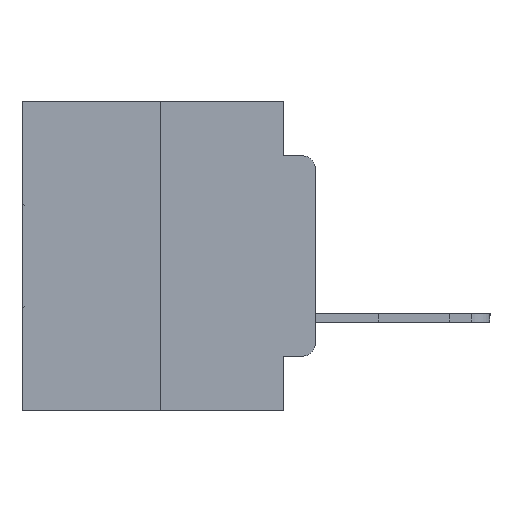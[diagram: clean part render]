
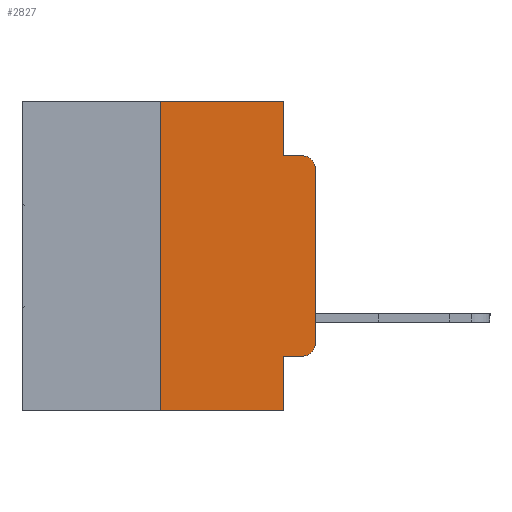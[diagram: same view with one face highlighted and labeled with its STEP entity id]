
A CAD part, left-side view. The second image highlights one B-rep face of the part: STEP entity #2827.
In plain terms, the highlighted planar face has unit normal (-1, 0, 0).
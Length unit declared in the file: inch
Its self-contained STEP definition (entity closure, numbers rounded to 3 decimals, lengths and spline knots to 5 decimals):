
#134 = CIRCLE ( 'NONE', #27930, 0.02 ) ;
#1123 = ORIENTED_EDGE ( 'NONE', *, *, #8856, .T. ) ;
#1332 = DIRECTION ( 'NONE',  ( 0., -1., 0. ) ) ;
#1491 = EDGE_CURVE ( 'NONE', #13249, #27975, #21771, .T. ) ;
#1554 = ORIENTED_EDGE ( 'NONE', *, *, #29062, .F. ) ;
#1798 = DIRECTION ( 'NONE',  ( 0., 0., -1. ) ) ;
#2827 = ADVANCED_FACE ( 'NONE', ( #18176 ), #4792, .F. ) ;
#3279 = EDGE_CURVE ( 'NONE', #28406, #4622, #22686, .T. ) ;
#3371 = CARTESIAN_POINT ( 'NONE',  ( 0., 0.051, 0. ) ) ;
#3413 = VECTOR ( 'NONE', #17441, 39.37008 ) ;
#3831 = VERTEX_POINT ( 'NONE', #18036 ) ;
#4171 = LINE ( 'NONE', #3371, #3413 ) ;
#4533 = CARTESIAN_POINT ( 'NONE',  ( 0., 0.25, 0. ) ) ;
#4622 = VERTEX_POINT ( 'NONE', #25711 ) ;
#4792 = PLANE ( 'NONE',  #17398 ) ;
#4821 = CARTESIAN_POINT ( 'NONE',  ( 0., 0.473, 0. ) ) ;
#4843 = EDGE_CURVE ( 'NONE', #28406, #24494, #4919, .T. ) ;
#4919 = LINE ( 'NONE', #4533, #10415 ) ;
#5857 = DIRECTION ( 'NONE',  ( 0., 0., -1. ) ) ;
#5871 = EDGE_CURVE ( 'NONE', #24494, #3831, #19081, .T. ) ;
#6150 = CARTESIAN_POINT ( 'NONE',  ( 0., 0.051, -0.4115 ) ) ;
#6652 = VECTOR ( 'NONE', #1332, 39.37008 ) ;
#7190 = DIRECTION ( 'NONE',  ( 0., -1., 0. ) ) ;
#7559 = ORIENTED_EDGE ( 'NONE', *, *, #9175, .T. ) ;
#7851 = DIRECTION ( 'NONE',  ( 0., 0., -1. ) ) ;
#7856 = DIRECTION ( 'NONE',  ( 1., 0., 0. ) ) ;
#8427 = LINE ( 'NONE', #21942, #13953 ) ;
#8856 = EDGE_CURVE ( 'NONE', #27269, #22256, #16182, .T. ) ;
#8903 = CARTESIAN_POINT ( 'NONE',  ( 0., 0., -0.3915 ) ) ;
#9065 = LINE ( 'NONE', #24958, #26474 ) ;
#9175 = EDGE_CURVE ( 'NONE', #22256, #16949, #134, .T. ) ;
#10415 = VECTOR ( 'NONE', #26581, 39.37008 ) ;
#10465 = VECTOR ( 'NONE', #12939, 39.37008 ) ;
#10766 = EDGE_CURVE ( 'NONE', #27975, #27269, #16026, .T. ) ;
#10768 = CARTESIAN_POINT ( 'NONE',  ( 0., 0.02, -0.3915 ) ) ;
#12939 = DIRECTION ( 'NONE',  ( 0., -1., 0. ) ) ;
#13145 = DIRECTION ( 'NONE',  ( 0., 0., -1. ) ) ;
#13249 = VERTEX_POINT ( 'NONE', #20065 ) ;
#13715 = DIRECTION ( 'NONE',  ( 0., -1., 0. ) ) ;
#13953 = VECTOR ( 'NONE', #5857, 39.37008 ) ;
#14979 = VECTOR ( 'NONE', #7190, 39.37008 ) ;
#15640 = ORIENTED_EDGE ( 'NONE', *, *, #1491, .T. ) ;
#15964 = CARTESIAN_POINT ( 'NONE',  ( 0., 0.02, -0.1085 ) ) ;
#16026 = CIRCLE ( 'NONE', #27968, 0.02 ) ;
#16182 = LINE ( 'NONE', #19670, #22228 ) ;
#16949 = VERTEX_POINT ( 'NONE', #23699 ) ;
#17398 = AXIS2_PLACEMENT_3D ( 'NONE', #4821, #7856, #7851 ) ;
#17441 = DIRECTION ( 'NONE',  ( 0., 0., -1. ) ) ;
#17458 = ORIENTED_EDGE ( 'NONE', *, *, #24851, .F. ) ;
#17580 = CARTESIAN_POINT ( 'NONE',  ( 0., 0.051, -0.0885 ) ) ;
#18036 = CARTESIAN_POINT ( 'NONE',  ( 0., 0.051, 0. ) ) ;
#18176 = FACE_OUTER_BOUND ( 'NONE', #28764, .T. ) ;
#18327 = DIRECTION ( 'NONE',  ( -1., 0., 0. ) ) ;
#18900 = ORIENTED_EDGE ( 'NONE', *, *, #4843, .F. ) ;
#19081 = LINE ( 'NONE', #28901, #6652 ) ;
#19670 = CARTESIAN_POINT ( 'NONE',  ( 0., 0., 0. ) ) ;
#20065 = CARTESIAN_POINT ( 'NONE',  ( 0., 0.051, -0.4115 ) ) ;
#21676 = CARTESIAN_POINT ( 'NONE',  ( 0., 0.25, 0. ) ) ;
#21771 = LINE ( 'NONE', #6150, #14979 ) ;
#21942 = CARTESIAN_POINT ( 'NONE',  ( 0., 0.051, 0. ) ) ;
#22228 = VECTOR ( 'NONE', #26869, 39.37008 ) ;
#22256 = VERTEX_POINT ( 'NONE', #23204 ) ;
#22686 = LINE ( 'NONE', #29485, #10465 ) ;
#22710 = CARTESIAN_POINT ( 'NONE',  ( 0., 0.02, -0.4115 ) ) ;
#23204 = CARTESIAN_POINT ( 'NONE',  ( 0., 0., -0.1085 ) ) ;
#23422 = ORIENTED_EDGE ( 'NONE', *, *, #5871, .F. ) ;
#23699 = CARTESIAN_POINT ( 'NONE',  ( 0., 0.02, -0.0885 ) ) ;
#24288 = CARTESIAN_POINT ( 'NONE',  ( 0., 0.25, -0.5 ) ) ;
#24494 = VERTEX_POINT ( 'NONE', #21676 ) ;
#24780 = ORIENTED_EDGE ( 'NONE', *, *, #3279, .T. ) ;
#24851 = EDGE_CURVE ( 'NONE', #3831, #25614, #8427, .T. ) ;
#24958 = CARTESIAN_POINT ( 'NONE',  ( 0., 0.051, -0.0885 ) ) ;
#25614 = VERTEX_POINT ( 'NONE', #17580 ) ;
#25711 = CARTESIAN_POINT ( 'NONE',  ( 0., 0.051, -0.5 ) ) ;
#25813 = EDGE_CURVE ( 'NONE', #25614, #16949, #9065, .T. ) ;
#26474 = VECTOR ( 'NONE', #13715, 39.37008 ) ;
#26581 = DIRECTION ( 'NONE',  ( 0., 0., 1. ) ) ;
#26602 = DIRECTION ( 'NONE',  ( -1., 0., 0. ) ) ;
#26869 = DIRECTION ( 'NONE',  ( 0., 0., 1. ) ) ;
#27141 = ORIENTED_EDGE ( 'NONE', *, *, #25813, .F. ) ;
#27269 = VERTEX_POINT ( 'NONE', #8903 ) ;
#27508 = ORIENTED_EDGE ( 'NONE', *, *, #10766, .T. ) ;
#27930 = AXIS2_PLACEMENT_3D ( 'NONE', #15964, #18327, #1798 ) ;
#27968 = AXIS2_PLACEMENT_3D ( 'NONE', #10768, #26602, #13145 ) ;
#27975 = VERTEX_POINT ( 'NONE', #22710 ) ;
#28406 = VERTEX_POINT ( 'NONE', #24288 ) ;
#28764 = EDGE_LOOP ( 'NONE', ( #1123, #7559, #27141, #17458, #23422, #18900, #24780, #1554, #15640, #27508 ) ) ;
#28901 = CARTESIAN_POINT ( 'NONE',  ( 0., 0.473, 0. ) ) ;
#29062 = EDGE_CURVE ( 'NONE', #13249, #4622, #4171, .T. ) ;
#29485 = CARTESIAN_POINT ( 'NONE',  ( 0., 0.473, -0.5 ) ) ;
